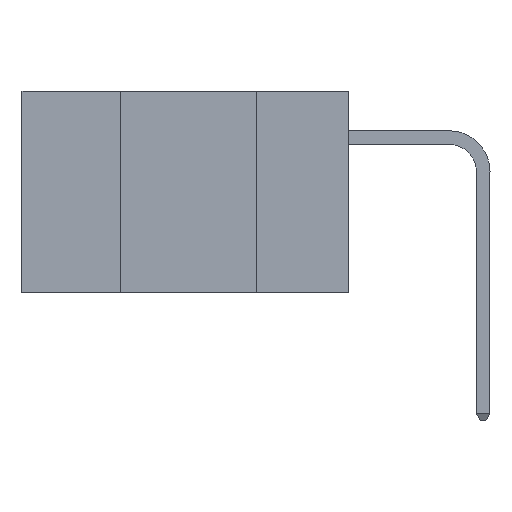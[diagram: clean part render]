
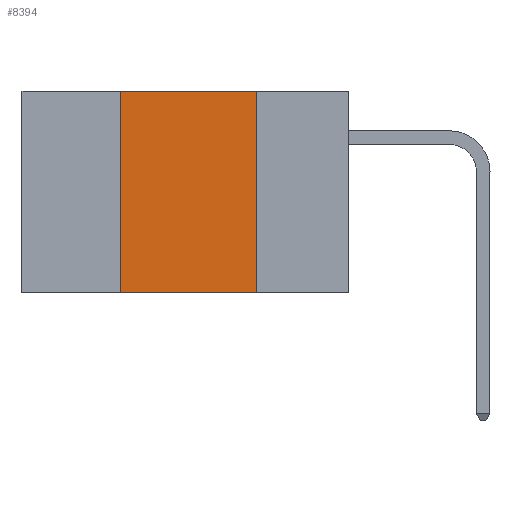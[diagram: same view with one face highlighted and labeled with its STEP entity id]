
A CAD part, left-side view. The second image highlights one B-rep face of the part: STEP entity #8394.
In plain terms, the highlighted planar face has unit normal (-1, 0, 0).
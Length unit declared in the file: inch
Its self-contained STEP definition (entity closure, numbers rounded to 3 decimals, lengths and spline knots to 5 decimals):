
#746 = AXIS2_PLACEMENT_3D ( 'NONE', #10868, #19876, #15548 ) ;
#862 = CARTESIAN_POINT ( 'NONE',  ( 0., 0.42, -0.37 ) ) ;
#1010 = EDGE_CURVE ( 'NONE', #21488, #19327, #7141, .T. ) ;
#1398 = EDGE_CURVE ( 'NONE', #11894, #21488, #26280, .T. ) ;
#1892 = ORIENTED_EDGE ( 'NONE', *, *, #11638, .T. ) ;
#4131 = FACE_OUTER_BOUND ( 'NONE', #28264, .T. ) ;
#5618 = CARTESIAN_POINT ( 'NONE',  ( 0., 0.6, 0. ) ) ;
#6144 = CARTESIAN_POINT ( 'NONE',  ( 0., 0.6, -0.37 ) ) ;
#6271 = CARTESIAN_POINT ( 'NONE',  ( 0., 0.17, 0. ) ) ;
#7141 = LINE ( 'NONE', #6271, #25950 ) ;
#7625 = ORIENTED_EDGE ( 'NONE', *, *, #1010, .F. ) ;
#8394 = ADVANCED_FACE ( 'NONE', ( #4131 ), #17737, .F. ) ;
#8819 = CARTESIAN_POINT ( 'NONE',  ( 0., 0.17, 0. ) ) ;
#10868 = CARTESIAN_POINT ( 'NONE',  ( 0., 0.6, 0. ) ) ;
#11100 = DIRECTION ( 'NONE',  ( 0., -1., 0. ) ) ;
#11638 = EDGE_CURVE ( 'NONE', #26906, #19327, #17627, .T. ) ;
#11683 = VECTOR ( 'NONE', #11100, 39.37008 ) ;
#11894 = VERTEX_POINT ( 'NONE', #19136 ) ;
#13403 = VECTOR ( 'NONE', #27787, 39.37008 ) ;
#15548 = DIRECTION ( 'NONE',  ( 0., 0., -1. ) ) ;
#16114 = CARTESIAN_POINT ( 'NONE',  ( 0., 0.17, -0.37 ) ) ;
#17092 = EDGE_CURVE ( 'NONE', #26906, #11894, #23933, .T. ) ;
#17265 = DIRECTION ( 'NONE',  ( 0., 0., -1. ) ) ;
#17627 = LINE ( 'NONE', #6144, #11683 ) ;
#17737 = PLANE ( 'NONE',  #746 ) ;
#19136 = CARTESIAN_POINT ( 'NONE',  ( 0., 0.42, 0. ) ) ;
#19327 = VERTEX_POINT ( 'NONE', #16114 ) ;
#19876 = DIRECTION ( 'NONE',  ( 1., 0., 0. ) ) ;
#21486 = VECTOR ( 'NONE', #28121, 39.37008 ) ;
#21488 = VERTEX_POINT ( 'NONE', #8819 ) ;
#21903 = CARTESIAN_POINT ( 'NONE',  ( 0., 0.42, 0. ) ) ;
#22469 = ORIENTED_EDGE ( 'NONE', *, *, #17092, .F. ) ;
#23933 = LINE ( 'NONE', #21903, #21486 ) ;
#24734 = ORIENTED_EDGE ( 'NONE', *, *, #1398, .F. ) ;
#25950 = VECTOR ( 'NONE', #17265, 39.37008 ) ;
#26280 = LINE ( 'NONE', #5618, #13403 ) ;
#26906 = VERTEX_POINT ( 'NONE', #862 ) ;
#27787 = DIRECTION ( 'NONE',  ( 0., -1., 0. ) ) ;
#28121 = DIRECTION ( 'NONE',  ( 0., 0., 1. ) ) ;
#28264 = EDGE_LOOP ( 'NONE', ( #7625, #24734, #22469, #1892 ) ) ;
